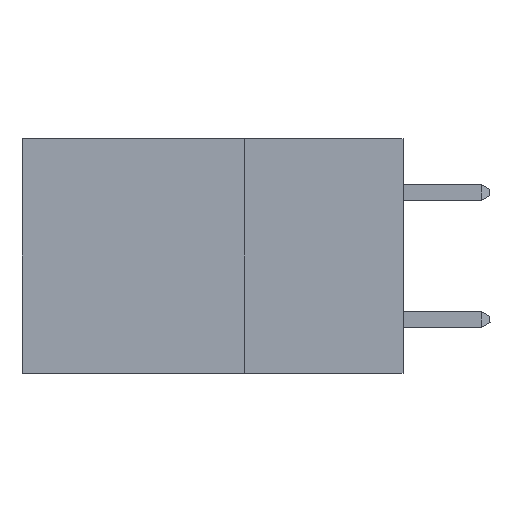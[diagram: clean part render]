
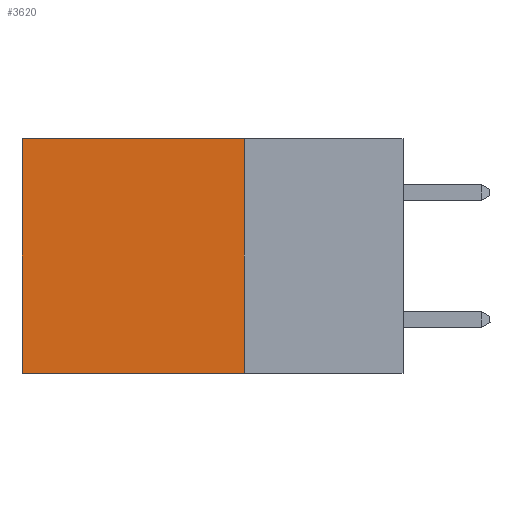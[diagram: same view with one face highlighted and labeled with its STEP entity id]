
A CAD part, left-side view. The second image highlights one B-rep face of the part: STEP entity #3620.
In plain terms, the highlighted planar face has unit normal (-1, 0, 0).
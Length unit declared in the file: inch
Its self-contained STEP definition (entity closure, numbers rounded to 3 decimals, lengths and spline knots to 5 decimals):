
#225 = VECTOR ( 'NONE', #11865, 39.37008 ) ;
#349 = ORIENTED_EDGE ( 'NONE', *, *, #12436, .F. ) ;
#756 = EDGE_LOOP ( 'NONE', ( #13098, #11608, #349, #772 ) ) ;
#772 = ORIENTED_EDGE ( 'NONE', *, *, #4299, .T. ) ;
#2027 = DIRECTION ( 'NONE',  ( 0., 0., -1. ) ) ;
#3470 = EDGE_CURVE ( 'NONE', #10594, #7202, #12834, .T. ) ;
#3620 = ADVANCED_FACE ( 'NONE', ( #12172 ), #5767, .F. ) ;
#3790 = CARTESIAN_POINT ( 'NONE',  ( 0.2875, 0.25, -0.37 ) ) ;
#4299 = EDGE_CURVE ( 'NONE', #13326, #10594, #5727, .T. ) ;
#4851 = DIRECTION ( 'NONE',  ( 0., 1., 0. ) ) ;
#5727 = LINE ( 'NONE', #9787, #225 ) ;
#5767 = PLANE ( 'NONE',  #8073 ) ;
#6501 = CARTESIAN_POINT ( 'NONE',  ( 0.2875, 0.25, -0.37 ) ) ;
#6672 = DIRECTION ( 'NONE',  ( 1., 0., 0. ) ) ;
#6774 = VECTOR ( 'NONE', #2027, 39.37008 ) ;
#7202 = VERTEX_POINT ( 'NONE', #11554 ) ;
#7569 = LINE ( 'NONE', #3790, #9642 ) ;
#7675 = VECTOR ( 'NONE', #12474, 39.37008 ) ;
#7705 = DIRECTION ( 'NONE',  ( 0., 0., -1. ) ) ;
#8073 = AXIS2_PLACEMENT_3D ( 'NONE', #12972, #6672, #7705 ) ;
#9258 = CARTESIAN_POINT ( 'NONE',  ( 0.2875, 0.25, 0. ) ) ;
#9642 = VECTOR ( 'NONE', #4851, 39.37008 ) ;
#9787 = CARTESIAN_POINT ( 'NONE',  ( 0.2875, 0.25, 0. ) ) ;
#10015 = VERTEX_POINT ( 'NONE', #6501 ) ;
#10399 = CARTESIAN_POINT ( 'NONE',  ( 0.2875, 0.6, 0. ) ) ;
#10594 = VERTEX_POINT ( 'NONE', #12582 ) ;
#11026 = EDGE_CURVE ( 'NONE', #10015, #7202, #7569, .T. ) ;
#11551 = CARTESIAN_POINT ( 'NONE',  ( 0.2875, 0.25, 0. ) ) ;
#11554 = CARTESIAN_POINT ( 'NONE',  ( 0.2875, 0.6, -0.37 ) ) ;
#11608 = ORIENTED_EDGE ( 'NONE', *, *, #11026, .F. ) ;
#11865 = DIRECTION ( 'NONE',  ( 0., 1., 0. ) ) ;
#12172 = FACE_OUTER_BOUND ( 'NONE', #756, .T. ) ;
#12436 = EDGE_CURVE ( 'NONE', #13326, #10015, #12904, .T. ) ;
#12474 = DIRECTION ( 'NONE',  ( 0., 0., -1. ) ) ;
#12582 = CARTESIAN_POINT ( 'NONE',  ( 0.2875, 0.6, 0. ) ) ;
#12834 = LINE ( 'NONE', #10399, #7675 ) ;
#12904 = LINE ( 'NONE', #9258, #6774 ) ;
#12972 = CARTESIAN_POINT ( 'NONE',  ( 0.2875, 0.25, 0. ) ) ;
#13098 = ORIENTED_EDGE ( 'NONE', *, *, #3470, .T. ) ;
#13326 = VERTEX_POINT ( 'NONE', #11551 ) ;
